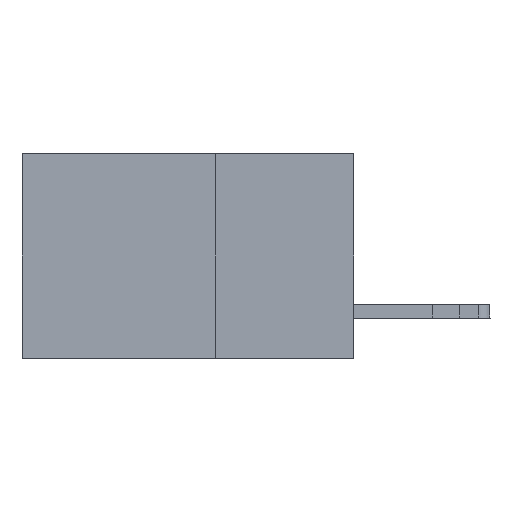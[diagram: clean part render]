
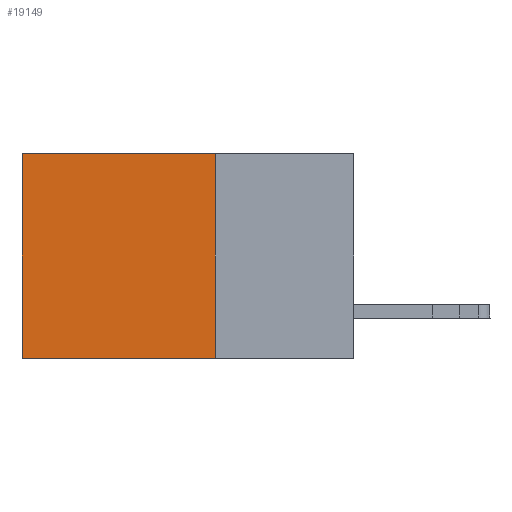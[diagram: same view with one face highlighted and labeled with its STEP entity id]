
A CAD part, left-side view. The second image highlights one B-rep face of the part: STEP entity #19149.
In plain terms, the highlighted planar face has unit normal (-1, 0, 0).
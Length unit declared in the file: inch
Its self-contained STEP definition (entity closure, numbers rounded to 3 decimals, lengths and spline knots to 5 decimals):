
#594 = VERTEX_POINT ( 'NONE', #1439 ) ;
#862 = CARTESIAN_POINT ( 'NONE',  ( 0.2875, 0.25, -0.37 ) ) ;
#982 = CARTESIAN_POINT ( 'NONE',  ( 0.2875, 0.6, -0.37 ) ) ;
#1093 = VECTOR ( 'NONE', #16851, 39.37008 ) ;
#1439 = CARTESIAN_POINT ( 'NONE',  ( 0.2875, 0.6, 0. ) ) ;
#1541 = VECTOR ( 'NONE', #10326, 39.37008 ) ;
#1544 = FACE_OUTER_BOUND ( 'NONE', #16349, .T. ) ;
#1709 = EDGE_CURVE ( 'NONE', #11607, #4741, #15747, .T. ) ;
#4187 = EDGE_CURVE ( 'NONE', #10642, #11607, #19571, .T. ) ;
#4741 = VERTEX_POINT ( 'NONE', #982 ) ;
#4799 = CARTESIAN_POINT ( 'NONE',  ( 0.2875, 0.25, 0. ) ) ;
#5022 = CARTESIAN_POINT ( 'NONE',  ( 0.2875, 0.6, 0. ) ) ;
#5168 = DIRECTION ( 'NONE',  ( 0., 1., 0. ) ) ;
#5327 = VECTOR ( 'NONE', #12751, 39.37008 ) ;
#7393 = VECTOR ( 'NONE', #5168, 39.37008 ) ;
#7841 = DIRECTION ( 'NONE',  ( 0., 0., -1. ) ) ;
#8436 = ORIENTED_EDGE ( 'NONE', *, *, #14869, .T. ) ;
#10326 = DIRECTION ( 'NONE',  ( 0., 1., 0. ) ) ;
#10421 = LINE ( 'NONE', #5022, #1093 ) ;
#10642 = VERTEX_POINT ( 'NONE', #20076 ) ;
#11607 = VERTEX_POINT ( 'NONE', #13837 ) ;
#12212 = CARTESIAN_POINT ( 'NONE',  ( 0.2875, 0.25, 0. ) ) ;
#12751 = DIRECTION ( 'NONE',  ( 0., 0., -1. ) ) ;
#13292 = ORIENTED_EDGE ( 'NONE', *, *, #18401, .T. ) ;
#13553 = ORIENTED_EDGE ( 'NONE', *, *, #4187, .F. ) ;
#13837 = CARTESIAN_POINT ( 'NONE',  ( 0.2875, 0.25, -0.37 ) ) ;
#14569 = ORIENTED_EDGE ( 'NONE', *, *, #1709, .F. ) ;
#14603 = CARTESIAN_POINT ( 'NONE',  ( 0.2875, 0.25, 0. ) ) ;
#14742 = AXIS2_PLACEMENT_3D ( 'NONE', #4799, #16528, #7841 ) ;
#14869 = EDGE_CURVE ( 'NONE', #594, #4741, #10421, .T. ) ;
#15275 = LINE ( 'NONE', #12212, #7393 ) ;
#15747 = LINE ( 'NONE', #862, #1541 ) ;
#16101 = PLANE ( 'NONE',  #14742 ) ;
#16349 = EDGE_LOOP ( 'NONE', ( #8436, #14569, #13553, #13292 ) ) ;
#16528 = DIRECTION ( 'NONE',  ( 1., 0., 0. ) ) ;
#16851 = DIRECTION ( 'NONE',  ( 0., 0., -1. ) ) ;
#18401 = EDGE_CURVE ( 'NONE', #10642, #594, #15275, .T. ) ;
#19149 = ADVANCED_FACE ( 'NONE', ( #1544 ), #16101, .F. ) ;
#19571 = LINE ( 'NONE', #14603, #5327 ) ;
#20076 = CARTESIAN_POINT ( 'NONE',  ( 0.2875, 0.25, 0. ) ) ;
